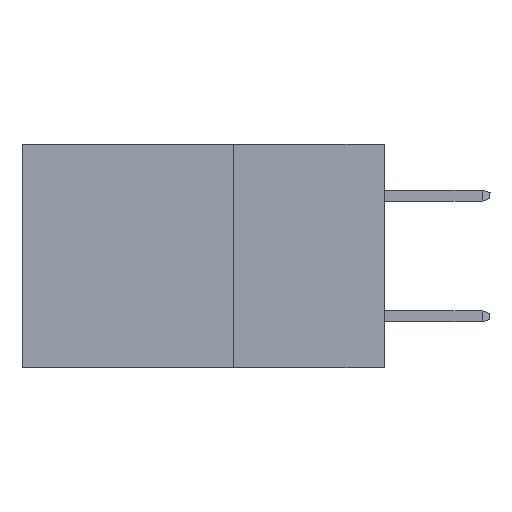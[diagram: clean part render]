
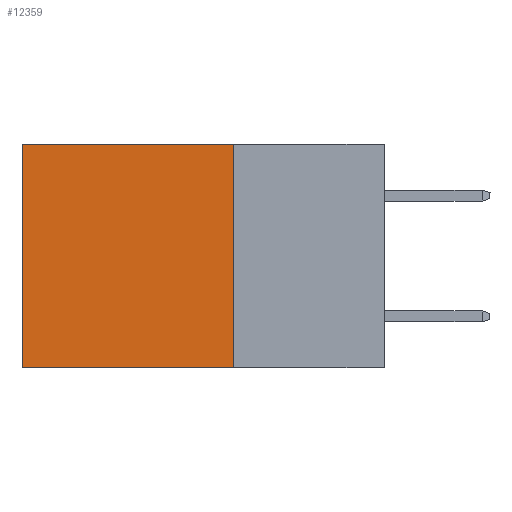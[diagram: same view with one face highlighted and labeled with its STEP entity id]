
A CAD part, left-side view. The second image highlights one B-rep face of the part: STEP entity #12359.
In plain terms, the highlighted planar face has unit normal (-1, 0, 0).
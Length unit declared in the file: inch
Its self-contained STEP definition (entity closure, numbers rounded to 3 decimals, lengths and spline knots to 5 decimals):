
#396 = LINE ( 'NONE', #31626, #24895 ) ;
#1425 = VERTEX_POINT ( 'NONE', #29747 ) ;
#1545 = DIRECTION ( 'NONE',  ( 0., 1., 0. ) ) ;
#3621 = EDGE_CURVE ( 'NONE', #27290, #28308, #18001, .T. ) ;
#4184 = LINE ( 'NONE', #19463, #13637 ) ;
#4265 = DIRECTION ( 'NONE',  ( 0., 1., 0. ) ) ;
#5584 = DIRECTION ( 'NONE',  ( 0., 0., -1. ) ) ;
#6915 = FACE_OUTER_BOUND ( 'NONE', #14490, .T. ) ;
#7922 = PLANE ( 'NONE',  #13398 ) ;
#10739 = CARTESIAN_POINT ( 'NONE',  ( 0.298, 0.25, 0. ) ) ;
#12359 = ADVANCED_FACE ( 'NONE', ( #6915 ), #7922, .F. ) ;
#12833 = CARTESIAN_POINT ( 'NONE',  ( 0.298, 0.6, -0.37 ) ) ;
#13398 = AXIS2_PLACEMENT_3D ( 'NONE', #25545, #20670, #5584 ) ;
#13637 = VECTOR ( 'NONE', #4265, 39.37008 ) ;
#14490 = EDGE_LOOP ( 'NONE', ( #27880, #21616, #19679, #15188 ) ) ;
#15188 = ORIENTED_EDGE ( 'NONE', *, *, #31987, .T. ) ;
#15651 = EDGE_CURVE ( 'NONE', #27020, #1425, #21281, .T. ) ;
#16953 = VECTOR ( 'NONE', #24445, 39.37008 ) ;
#18001 = LINE ( 'NONE', #22483, #32563 ) ;
#19463 = CARTESIAN_POINT ( 'NONE',  ( 0.298, 0.25, -0.37 ) ) ;
#19679 = ORIENTED_EDGE ( 'NONE', *, *, #15651, .F. ) ;
#20670 = DIRECTION ( 'NONE',  ( 1., 0., 0. ) ) ;
#21022 = EDGE_CURVE ( 'NONE', #1425, #28308, #4184, .T. ) ;
#21281 = LINE ( 'NONE', #31908, #16953 ) ;
#21616 = ORIENTED_EDGE ( 'NONE', *, *, #21022, .F. ) ;
#22483 = CARTESIAN_POINT ( 'NONE',  ( 0.298, 0.6, 0. ) ) ;
#24445 = DIRECTION ( 'NONE',  ( 0., 0., -1. ) ) ;
#24895 = VECTOR ( 'NONE', #1545, 39.37008 ) ;
#25029 = CARTESIAN_POINT ( 'NONE',  ( 0.298, 0.6, 0. ) ) ;
#25545 = CARTESIAN_POINT ( 'NONE',  ( 0.298, 0.25, 0. ) ) ;
#27020 = VERTEX_POINT ( 'NONE', #10739 ) ;
#27290 = VERTEX_POINT ( 'NONE', #25029 ) ;
#27880 = ORIENTED_EDGE ( 'NONE', *, *, #3621, .T. ) ;
#28308 = VERTEX_POINT ( 'NONE', #12833 ) ;
#29747 = CARTESIAN_POINT ( 'NONE',  ( 0.298, 0.25, -0.37 ) ) ;
#30404 = DIRECTION ( 'NONE',  ( 0., 0., -1. ) ) ;
#31626 = CARTESIAN_POINT ( 'NONE',  ( 0.298, 0.25, 0. ) ) ;
#31908 = CARTESIAN_POINT ( 'NONE',  ( 0.298, 0.25, 0. ) ) ;
#31987 = EDGE_CURVE ( 'NONE', #27020, #27290, #396, .T. ) ;
#32563 = VECTOR ( 'NONE', #30404, 39.37008 ) ;
